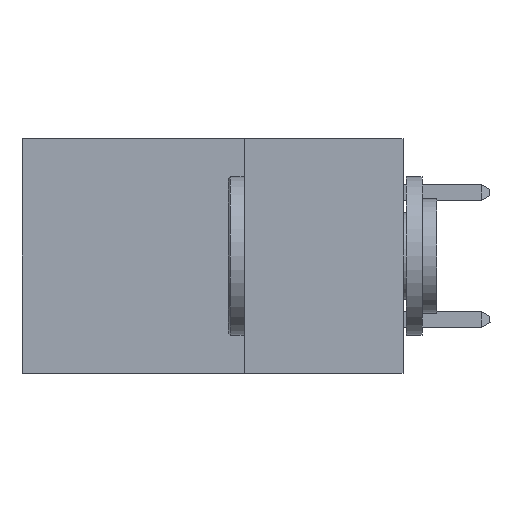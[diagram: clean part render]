
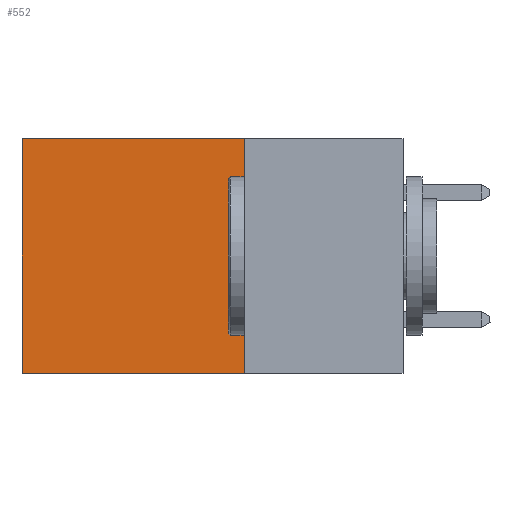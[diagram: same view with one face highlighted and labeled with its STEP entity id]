
A CAD part, left-side view. The second image highlights one B-rep face of the part: STEP entity #552.
In plain terms, the highlighted planar face has unit normal (-1, 0, 0).
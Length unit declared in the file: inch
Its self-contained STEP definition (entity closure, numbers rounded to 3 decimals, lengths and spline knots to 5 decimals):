
#282 = CARTESIAN_POINT ( 'NONE',  ( 0.2875, 0.25, 0. ) ) ;
#542 = PLANE ( 'NONE',  #12879 ) ;
#552 = ADVANCED_FACE ( 'NONE', ( #18549 ), #542, .F. ) ;
#1179 = EDGE_CURVE ( 'NONE', #1779, #19132, #15021, .T. ) ;
#1779 = VERTEX_POINT ( 'NONE', #3372 ) ;
#1829 = DIRECTION ( 'NONE',  ( 0., 0., -1. ) ) ;
#1916 = DIRECTION ( 'NONE',  ( 1., 0., 0. ) ) ;
#2009 = CARTESIAN_POINT ( 'NONE',  ( 0.2875, 0.6, 0. ) ) ;
#3372 = CARTESIAN_POINT ( 'NONE',  ( 0.2875, 0.25, -0.37 ) ) ;
#3764 = DIRECTION ( 'NONE',  ( 0., 0., -1. ) ) ;
#3889 = LINE ( 'NONE', #15129, #18334 ) ;
#4904 = EDGE_LOOP ( 'NONE', ( #20248, #14916, #10164, #7979 ) ) ;
#5872 = CARTESIAN_POINT ( 'NONE',  ( 0.2875, 0.25, -0.37 ) ) ;
#6881 = DIRECTION ( 'NONE',  ( 0., 1., 0. ) ) ;
#7979 = ORIENTED_EDGE ( 'NONE', *, *, #16660, .T. ) ;
#10164 = ORIENTED_EDGE ( 'NONE', *, *, #16351, .F. ) ;
#11511 = LINE ( 'NONE', #20071, #12115 ) ;
#12115 = VECTOR ( 'NONE', #6881, 39.37008 ) ;
#12879 = AXIS2_PLACEMENT_3D ( 'NONE', #22120, #1916, #15978 ) ;
#13623 = LINE ( 'NONE', #15099, #18600 ) ;
#14916 = ORIENTED_EDGE ( 'NONE', *, *, #1179, .F. ) ;
#15021 = LINE ( 'NONE', #5872, #24534 ) ;
#15099 = CARTESIAN_POINT ( 'NONE',  ( 0.2875, 0.25, 0. ) ) ;
#15129 = CARTESIAN_POINT ( 'NONE',  ( 0.2875, 0.6, 0. ) ) ;
#15728 = EDGE_CURVE ( 'NONE', #24139, #19132, #3889, .T. ) ;
#15978 = DIRECTION ( 'NONE',  ( 0., 0., -1. ) ) ;
#16351 = EDGE_CURVE ( 'NONE', #18577, #1779, #13623, .T. ) ;
#16660 = EDGE_CURVE ( 'NONE', #18577, #24139, #11511, .T. ) ;
#18334 = VECTOR ( 'NONE', #1829, 39.37008 ) ;
#18549 = FACE_OUTER_BOUND ( 'NONE', #4904, .T. ) ;
#18577 = VERTEX_POINT ( 'NONE', #282 ) ;
#18600 = VECTOR ( 'NONE', #3764, 39.37008 ) ;
#19132 = VERTEX_POINT ( 'NONE', #22537 ) ;
#20071 = CARTESIAN_POINT ( 'NONE',  ( 0.2875, 0.25, 0. ) ) ;
#20248 = ORIENTED_EDGE ( 'NONE', *, *, #15728, .T. ) ;
#22120 = CARTESIAN_POINT ( 'NONE',  ( 0.2875, 0.25, 0. ) ) ;
#22537 = CARTESIAN_POINT ( 'NONE',  ( 0.2875, 0.6, -0.37 ) ) ;
#23190 = DIRECTION ( 'NONE',  ( 0., 1., 0. ) ) ;
#24139 = VERTEX_POINT ( 'NONE', #2009 ) ;
#24534 = VECTOR ( 'NONE', #23190, 39.37008 ) ;
